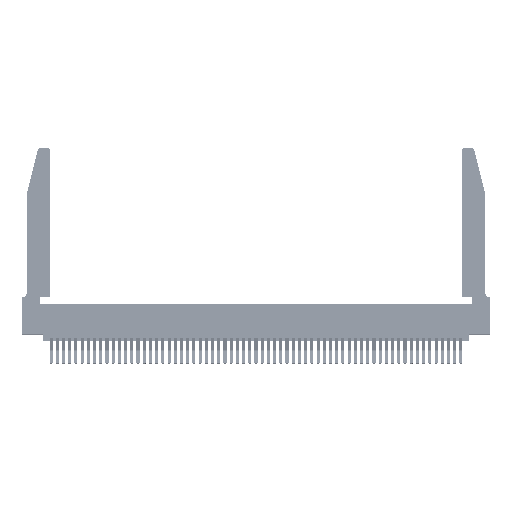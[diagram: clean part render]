
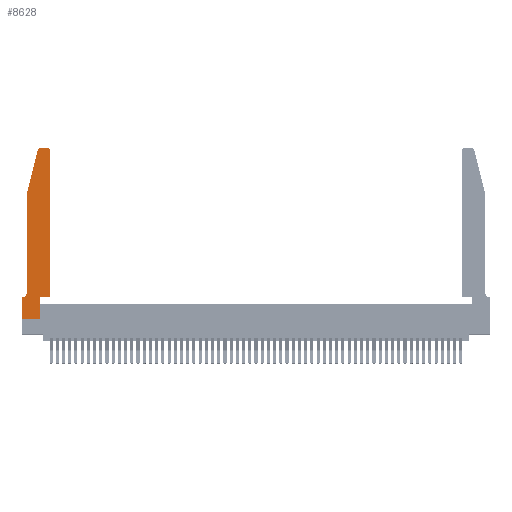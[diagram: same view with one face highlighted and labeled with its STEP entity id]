
A CAD part, top view. The second image highlights one B-rep face of the part: STEP entity #8628.
In plain terms, the highlighted planar face has unit normal (0, 0, 1).
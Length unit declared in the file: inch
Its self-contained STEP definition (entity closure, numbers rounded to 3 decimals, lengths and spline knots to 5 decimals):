
#304 = CARTESIAN_POINT ( 'NONE',  ( 0.25487, 2.72718, 0.37 ) ) ;
#410 = ORIENTED_EDGE ( 'NONE', *, *, #23755, .T. ) ;
#825 = ORIENTED_EDGE ( 'NONE', *, *, #42139, .T. ) ;
#1101 = PLANE ( 'NONE',  #20502 ) ;
#1287 = AXIS2_PLACEMENT_3D ( 'NONE', #31242, #6158, #35475 ) ;
#1715 = VECTOR ( 'NONE', #34438, 39.37008 ) ;
#1722 = VERTEX_POINT ( 'NONE', #43376 ) ;
#1957 = CIRCLE ( 'NONE', #17719, 0.03 ) ;
#3120 = CARTESIAN_POINT ( 'NONE',  ( 0., 0., 0.37 ) ) ;
#3631 = LINE ( 'NONE', #22350, #34505 ) ;
#4325 = VERTEX_POINT ( 'NONE', #18250 ) ;
#4698 = CARTESIAN_POINT ( 'NONE',  ( 0.4505, 2.72, 0.37 ) ) ;
#4787 = LINE ( 'NONE', #16506, #6122 ) ;
#5169 = ORIENTED_EDGE ( 'NONE', *, *, #32124, .T. ) ;
#5544 = CARTESIAN_POINT ( 'NONE',  ( 0.284, 2.72, 0.37 ) ) ;
#5903 = VECTOR ( 'NONE', #33663, 39.37008 ) ;
#6122 = VECTOR ( 'NONE', #33339, 39.37008 ) ;
#6158 = DIRECTION ( 'NONE',  ( 0., 0., -1. ) ) ;
#7062 = VERTEX_POINT ( 'NONE', #4698 ) ;
#7714 = ORIENTED_EDGE ( 'NONE', *, *, #49719, .T. ) ;
#8217 = ORIENTED_EDGE ( 'NONE', *, *, #48357, .T. ) ;
#8628 = ADVANCED_FACE ( 'NONE', ( #11903 ), #1101, .T. ) ;
#8654 = EDGE_CURVE ( 'NONE', #29386, #26390, #1957, .T. ) ;
#9138 = EDGE_CURVE ( 'NONE', #48486, #1722, #11854, .T. ) ;
#9583 = ORIENTED_EDGE ( 'NONE', *, *, #32036, .T. ) ;
#9589 = DIRECTION ( 'NONE',  ( 0., 0., 1. ) ) ;
#9767 = DIRECTION ( 'NONE',  ( 1., 0., 0. ) ) ;
#9795 = VERTEX_POINT ( 'NONE', #25033 ) ;
#11144 = VECTOR ( 'NONE', #35625, 39.37008 ) ;
#11293 = VERTEX_POINT ( 'NONE', #48856 ) ;
#11564 = CIRCLE ( 'NONE', #1287, 0.07 ) ;
#11617 = EDGE_CURVE ( 'NONE', #17913, #4325, #12983, .T. ) ;
#11854 = LINE ( 'NONE', #20919, #21638 ) ;
#11894 = CARTESIAN_POINT ( 'NONE',  ( 0.0755, 2., 0.37 ) ) ;
#11903 = FACE_OUTER_BOUND ( 'NONE', #26553, .T. ) ;
#12144 = AXIS2_PLACEMENT_3D ( 'NONE', #41542, #16474, #45748 ) ;
#12796 = DIRECTION ( 'NONE',  ( -0.239, -0.971, 0. ) ) ;
#12864 = ORIENTED_EDGE ( 'NONE', *, *, #11617, .T. ) ;
#12983 = LINE ( 'NONE', #42653, #1715 ) ;
#16474 = DIRECTION ( 'NONE',  ( 0., 0., 1. ) ) ;
#16506 = CARTESIAN_POINT ( 'NONE',  ( 0., 0., 0.37 ) ) ;
#17719 = AXIS2_PLACEMENT_3D ( 'NONE', #5544, #34893, #9767 ) ;
#17913 = VERTEX_POINT ( 'NONE', #27594 ) ;
#18250 = CARTESIAN_POINT ( 'NONE',  ( 0.4505, 0.35, 0.37 ) ) ;
#18565 = CARTESIAN_POINT ( 'NONE',  ( 0.0755, 0.42, 0.37 ) ) ;
#19046 = VERTEX_POINT ( 'NONE', #18565 ) ;
#20502 = AXIS2_PLACEMENT_3D ( 'NONE', #34713, #9589, #38905 ) ;
#20919 = CARTESIAN_POINT ( 'NONE',  ( 0., 0., 0.37 ) ) ;
#20989 = ORIENTED_EDGE ( 'NONE', *, *, #35406, .T. ) ;
#21003 = CARTESIAN_POINT ( 'NONE',  ( 0.4505, 0.35, 0.37 ) ) ;
#21626 = LINE ( 'NONE', #30105, #42602 ) ;
#21638 = VECTOR ( 'NONE', #29314, 39.37008 ) ;
#22265 = LINE ( 'NONE', #31393, #11144 ) ;
#22350 = CARTESIAN_POINT ( 'NONE',  ( 0.2865, 0.35, 0.37 ) ) ;
#23755 = EDGE_CURVE ( 'NONE', #52277, #48486, #4787, .T. ) ;
#25033 = CARTESIAN_POINT ( 'NONE',  ( 0.0055, 0.35, 0.37 ) ) ;
#26390 = VERTEX_POINT ( 'NONE', #304 ) ;
#26553 = EDGE_LOOP ( 'NONE', ( #5169, #53217, #52263, #40565, #825, #8217, #410, #31257, #20989, #12864, #9583, #7714 ) ) ;
#26920 = VECTOR ( 'NONE', #12796, 39.37008 ) ;
#27529 = DIRECTION ( 'NONE',  ( -1., 0., 0. ) ) ;
#27594 = CARTESIAN_POINT ( 'NONE',  ( 0.2865, 0.35, 0.37 ) ) ;
#28822 = CARTESIAN_POINT ( 'NONE',  ( 0., 0.35, 0.37 ) ) ;
#29314 = DIRECTION ( 'NONE',  ( 1., 0., 0. ) ) ;
#29386 = VERTEX_POINT ( 'NONE', #40513 ) ;
#30105 = CARTESIAN_POINT ( 'NONE',  ( 0.2605, 2.75, 0.37 ) ) ;
#30755 = CIRCLE ( 'NONE', #12144, 0.03 ) ;
#31242 = CARTESIAN_POINT ( 'NONE',  ( 0.0055, 0.42, 0.37 ) ) ;
#31257 = ORIENTED_EDGE ( 'NONE', *, *, #9138, .T. ) ;
#31393 = CARTESIAN_POINT ( 'NONE',  ( 0.0755, 2., 0.37 ) ) ;
#32036 = EDGE_CURVE ( 'NONE', #4325, #7062, #38050, .T. ) ;
#32124 = EDGE_CURVE ( 'NONE', #11293, #29386, #21626, .T. ) ;
#32367 = EDGE_CURVE ( 'NONE', #49694, #19046, #22265, .T. ) ;
#33339 = DIRECTION ( 'NONE',  ( 0., -1., 0. ) ) ;
#33663 = DIRECTION ( 'NONE',  ( 0., 1., 0. ) ) ;
#34377 = DIRECTION ( 'NONE',  ( -1., 0., 0. ) ) ;
#34438 = DIRECTION ( 'NONE',  ( 1., 0., 0. ) ) ;
#34505 = VECTOR ( 'NONE', #47423, 39.37008 ) ;
#34713 = CARTESIAN_POINT ( 'NONE',  ( 0., 0.35, 0.37 ) ) ;
#34893 = DIRECTION ( 'NONE',  ( 0., 0., 1. ) ) ;
#35406 = EDGE_CURVE ( 'NONE', #1722, #17913, #3631, .T. ) ;
#35475 = DIRECTION ( 'NONE',  ( -1., 0., 0. ) ) ;
#35625 = DIRECTION ( 'NONE',  ( 0., -1., 0. ) ) ;
#38050 = LINE ( 'NONE', #21003, #5903 ) ;
#38905 = DIRECTION ( 'NONE',  ( 1., 0., 0. ) ) ;
#40027 = CARTESIAN_POINT ( 'NONE',  ( 0.0755, 0.35, 0.37 ) ) ;
#40513 = CARTESIAN_POINT ( 'NONE',  ( 0.284, 2.75, 0.37 ) ) ;
#40565 = ORIENTED_EDGE ( 'NONE', *, *, #32367, .T. ) ;
#40707 = VECTOR ( 'NONE', #27529, 39.37008 ) ;
#41542 = CARTESIAN_POINT ( 'NONE',  ( 0.4205, 2.72, 0.37 ) ) ;
#42064 = CARTESIAN_POINT ( 'NONE',  ( 0.0755, 2., 0.37 ) ) ;
#42139 = EDGE_CURVE ( 'NONE', #19046, #9795, #11564, .T. ) ;
#42602 = VECTOR ( 'NONE', #34377, 39.37008 ) ;
#42653 = CARTESIAN_POINT ( 'NONE',  ( 0.4505, 0.35, 0.37 ) ) ;
#43376 = CARTESIAN_POINT ( 'NONE',  ( 0.2865, 0., 0.37 ) ) ;
#45748 = DIRECTION ( 'NONE',  ( 1., 0., 0. ) ) ;
#47423 = DIRECTION ( 'NONE',  ( 0., 1., 0. ) ) ;
#47894 = LINE ( 'NONE', #42064, #26920 ) ;
#48021 = EDGE_CURVE ( 'NONE', #26390, #49694, #47894, .T. ) ;
#48357 = EDGE_CURVE ( 'NONE', #9795, #52277, #53049, .T. ) ;
#48486 = VERTEX_POINT ( 'NONE', #3120 ) ;
#48856 = CARTESIAN_POINT ( 'NONE',  ( 0.4205, 2.75, 0.37 ) ) ;
#49694 = VERTEX_POINT ( 'NONE', #11894 ) ;
#49719 = EDGE_CURVE ( 'NONE', #7062, #11293, #30755, .T. ) ;
#52263 = ORIENTED_EDGE ( 'NONE', *, *, #48021, .T. ) ;
#52277 = VERTEX_POINT ( 'NONE', #28822 ) ;
#53049 = LINE ( 'NONE', #40027, #40707 ) ;
#53217 = ORIENTED_EDGE ( 'NONE', *, *, #8654, .T. ) ;
